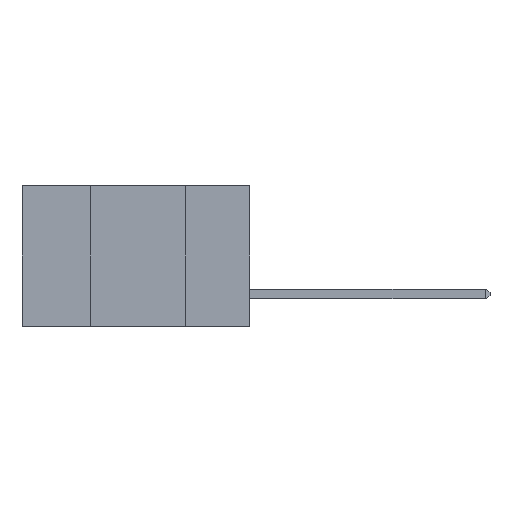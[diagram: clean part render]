
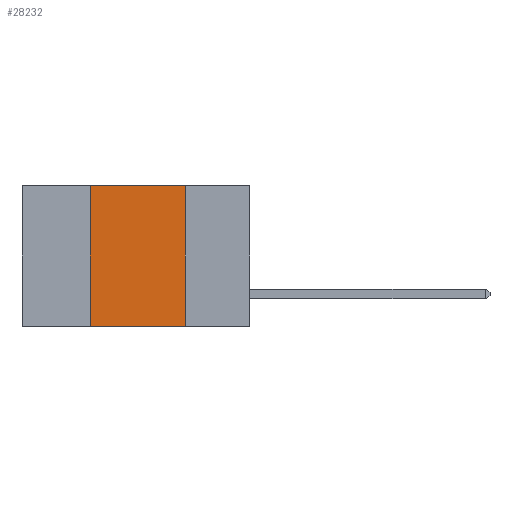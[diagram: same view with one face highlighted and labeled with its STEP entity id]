
A CAD part, left-side view. The second image highlights one B-rep face of the part: STEP entity #28232.
In plain terms, the highlighted planar face has unit normal (-1, 0, 0).
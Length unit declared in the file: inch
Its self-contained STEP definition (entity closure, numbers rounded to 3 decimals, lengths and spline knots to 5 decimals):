
#3329 = PLANE ( 'NONE',  #27050 ) ;
#5410 = VECTOR ( 'NONE', #16638, 39.37008 ) ;
#5723 = LINE ( 'NONE', #28451, #20422 ) ;
#6345 = DIRECTION ( 'NONE',  ( 1., 0., 0. ) ) ;
#7313 = EDGE_LOOP ( 'NONE', ( #13696, #35040, #35445, #19905 ) ) ;
#7929 = CARTESIAN_POINT ( 'NONE',  ( 0., 0.6, -0.37 ) ) ;
#8310 = VERTEX_POINT ( 'NONE', #35320 ) ;
#10756 = DIRECTION ( 'NONE',  ( 0., 0., -1. ) ) ;
#10888 = CARTESIAN_POINT ( 'NONE',  ( 0., 0.17, 0. ) ) ;
#12283 = EDGE_CURVE ( 'NONE', #36417, #25297, #20994, .T. ) ;
#13646 = CARTESIAN_POINT ( 'NONE',  ( 0., 0.6, 0. ) ) ;
#13696 = ORIENTED_EDGE ( 'NONE', *, *, #15418, .F. ) ;
#14101 = CARTESIAN_POINT ( 'NONE',  ( 0., 0.42, 0. ) ) ;
#15418 = EDGE_CURVE ( 'NONE', #8310, #25297, #24278, .T. ) ;
#16181 = LINE ( 'NONE', #13646, #23129 ) ;
#16458 = VECTOR ( 'NONE', #10756, 39.37008 ) ;
#16638 = DIRECTION ( 'NONE',  ( 0., -1., 0. ) ) ;
#17996 = CARTESIAN_POINT ( 'NONE',  ( 0., 0.6, 0. ) ) ;
#19905 = ORIENTED_EDGE ( 'NONE', *, *, #12283, .T. ) ;
#20422 = VECTOR ( 'NONE', #31305, 39.37008 ) ;
#20994 = LINE ( 'NONE', #7929, #5410 ) ;
#21637 = CARTESIAN_POINT ( 'NONE',  ( 0., 0.17, -0.37 ) ) ;
#23118 = EDGE_CURVE ( 'NONE', #35394, #8310, #16181, .T. ) ;
#23129 = VECTOR ( 'NONE', #28427, 39.37008 ) ;
#24278 = LINE ( 'NONE', #10888, #16458 ) ;
#25297 = VERTEX_POINT ( 'NONE', #21637 ) ;
#26456 = CARTESIAN_POINT ( 'NONE',  ( 0., 0.42, -0.37 ) ) ;
#26859 = DIRECTION ( 'NONE',  ( 0., 0., -1. ) ) ;
#27050 = AXIS2_PLACEMENT_3D ( 'NONE', #17996, #6345, #26859 ) ;
#28232 = ADVANCED_FACE ( 'NONE', ( #29030 ), #3329, .F. ) ;
#28427 = DIRECTION ( 'NONE',  ( 0., -1., 0. ) ) ;
#28451 = CARTESIAN_POINT ( 'NONE',  ( 0., 0.42, 0. ) ) ;
#29030 = FACE_OUTER_BOUND ( 'NONE', #7313, .T. ) ;
#31305 = DIRECTION ( 'NONE',  ( 0., 0., 1. ) ) ;
#35040 = ORIENTED_EDGE ( 'NONE', *, *, #23118, .F. ) ;
#35320 = CARTESIAN_POINT ( 'NONE',  ( 0., 0.17, 0. ) ) ;
#35394 = VERTEX_POINT ( 'NONE', #14101 ) ;
#35445 = ORIENTED_EDGE ( 'NONE', *, *, #35999, .F. ) ;
#35999 = EDGE_CURVE ( 'NONE', #36417, #35394, #5723, .T. ) ;
#36417 = VERTEX_POINT ( 'NONE', #26456 ) ;
